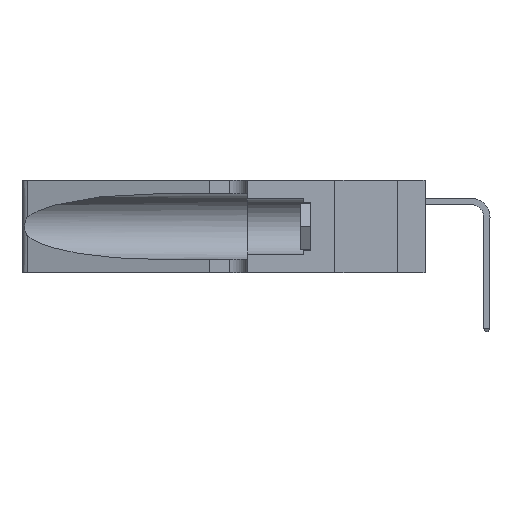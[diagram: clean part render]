
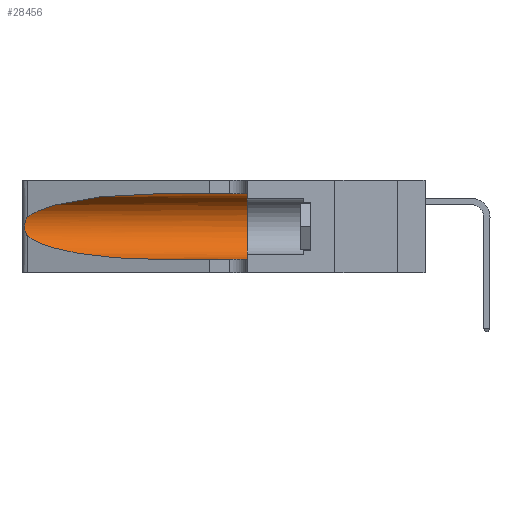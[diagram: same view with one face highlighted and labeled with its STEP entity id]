
A CAD part, left-side view. The second image highlights one B-rep face of the part: STEP entity #28456.
In plain terms, the highlighted cylindrical face has radius 3.308 mm (diameter 6.617 mm), a partial arc.
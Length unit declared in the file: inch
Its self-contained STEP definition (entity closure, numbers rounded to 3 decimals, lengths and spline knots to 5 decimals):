
#971 = CARTESIAN_POINT ( 'NONE',  ( 0.25787, 1.23484, 0.2124 ) ) ;
#2209 = CARTESIAN_POINT ( 'NONE',  ( 0.1305, 0.72297, 0.31525 ) ) ;
#2385 = B_SPLINE_CURVE_WITH_KNOTS ( 'NONE', 3,
 ( #15900, #33694, #18909, #971, #21850, #4006, #24819, #6992, #27801, #10040, #30830, #13051, #33829, #16030 ),
 .UNSPECIFIED., .F., .F.,
 ( 4, 2, 2, 2, 2, 2, 4 ),
 ( 0., 0.00027, 0.00053, 0.00107, 0.0016, 0.00187, 0.00214 ),
 .UNSPECIFIED. ) ;
#4006 = CARTESIAN_POINT ( 'NONE',  ( 0.26018, 1.23835, 0.19895 ) ) ;
#4031 = CYLINDRICAL_SURFACE ( 'NONE', #36166, 0.13025 ) ;
#4401 = CARTESIAN_POINT ( 'NONE',  ( 0.1305, 1.61858, 0.31525 ) ) ;
#5489 = VECTOR ( 'NONE', #11090, 39.37008 ) ;
#5728 = CARTESIAN_POINT ( 'NONE',  ( 0.1305, 0.35, 0.31525 ) ) ;
#6696 = CARTESIAN_POINT ( 'NONE',  ( 0.25487, 1.22718, 0.14631 ) ) ;
#6992 = CARTESIAN_POINT ( 'NONE',  ( 0.26075, 1.23896, 0.178 ) ) ;
#7516 = CARTESIAN_POINT ( 'NONE',  ( 0.18966, 0.96281, 0.31525 ) ) ;
#8796 = ORIENTED_EDGE ( 'NONE', *, *, #12495, .F. ) ;
#9128 = ORIENTED_EDGE ( 'NONE', *, *, #11429, .T. ) ;
#9142 = DIRECTION ( 'NONE',  ( 0., 1., 0. ) ) ;
#9740 = CARTESIAN_POINT ( 'NONE',  ( 0.2373, 1.15595, 0.08982 ) ) ;
#10040 = CARTESIAN_POINT ( 'NONE',  ( 0.25856, 1.23593, 0.16098 ) ) ;
#10431 = ORIENTED_EDGE ( 'NONE', *, *, #27737, .T. ) ;
#11090 = DIRECTION ( 'NONE',  ( 0., -1., 0. ) ) ;
#11429 = EDGE_CURVE ( 'NONE', #23252, #27129, #22519, .T. ) ;
#12495 = EDGE_CURVE ( 'NONE', #16182, #30165, #17047, .T. ) ;
#12679 = CARTESIAN_POINT ( 'NONE',  ( 0.1305, 0.35, 0.05475 ) ) ;
#12764 = CARTESIAN_POINT ( 'NONE',  ( 0.1305, 0.72297, 0.05475 ) ) ;
#13051 = CARTESIAN_POINT ( 'NONE',  ( 0.25639, 1.23186, 0.15144 ) ) ;
#13480 = LINE ( 'NONE', #22896, #5489 ) ;
#13501 = LINE ( 'NONE', #4401, #20459 ) ;
#13576 = CARTESIAN_POINT ( 'NONE',  ( 0.1305, 0.72297, 0.31525 ) ) ;
#14316 = DIRECTION ( 'NONE',  ( 0., -1., 0. ) ) ;
#15900 = CARTESIAN_POINT ( 'NONE',  ( 0.25487, 1.22718, 0.22369 ) ) ;
#16030 = CARTESIAN_POINT ( 'NONE',  ( 0.25487, 1.22718, 0.14631 ) ) ;
#16182 = VERTEX_POINT ( 'NONE', #5728 ) ;
#16577 = EDGE_CURVE ( 'NONE', #23252, #16182, #13501, .T. ) ;
#17047 = CIRCLE ( 'NONE', #26182, 0.13025 ) ;
#18909 = CARTESIAN_POINT ( 'NONE',  ( 0.25639, 1.23184, 0.21858 ) ) ;
#20259 = VERTEX_POINT ( 'NONE', #22179 ) ;
#20459 = VECTOR ( 'NONE', #28189, 39.37008 ) ;
#20836 = FACE_OUTER_BOUND ( 'NONE', #25506, .T. ) ;
#21850 = CARTESIAN_POINT ( 'NONE',  ( 0.25854, 1.2359, 0.20912 ) ) ;
#22179 = CARTESIAN_POINT ( 'NONE',  ( 0.1305, 0.72297, 0.05475 ) ) ;
#22519 =( BOUNDED_CURVE ( )  B_SPLINE_CURVE ( 3, ( #13576, #7516, #25333, #34333 ),
 .UNSPECIFIED., .F., .F. ) 
 B_SPLINE_CURVE_WITH_KNOTS ( ( 4, 4 ),
 ( 1.5708, 2.84003 ),
 .UNSPECIFIED. ) 
 CURVE ( )  GEOMETRIC_REPRESENTATION_ITEM ( )  RATIONAL_B_SPLINE_CURVE ( ( 1., 0.87, 0.87, 1. ) ) 
 REPRESENTATION_ITEM ( '' )  );
#22896 = CARTESIAN_POINT ( 'NONE',  ( 0.1305, 1.61858, 0.05475 ) ) ;
#23188 =( BOUNDED_CURVE ( )  B_SPLINE_CURVE ( 3, ( #6696, #9740, #30521, #12764 ),
 .UNSPECIFIED., .F., .F. ) 
 B_SPLINE_CURVE_WITH_KNOTS ( ( 4, 4 ),
 ( 3.44316, 4.71239 ),
 .UNSPECIFIED. ) 
 CURVE ( )  GEOMETRIC_REPRESENTATION_ITEM ( )  RATIONAL_B_SPLINE_CURVE ( ( 1., 0.87, 0.87, 1. ) ) 
 REPRESENTATION_ITEM ( '' )  );
#23252 = VERTEX_POINT ( 'NONE', #2209 ) ;
#23582 = EDGE_CURVE ( 'NONE', #32000, #20259, #23188, .T. ) ;
#24819 = CARTESIAN_POINT ( 'NONE',  ( 0.26075, 1.23896, 0.19203 ) ) ;
#25007 = EDGE_CURVE ( 'NONE', #27129, #32000, #2385, .T. ) ;
#25333 = CARTESIAN_POINT ( 'NONE',  ( 0.2373, 1.15595, 0.28018 ) ) ;
#25506 = EDGE_LOOP ( 'NONE', ( #9128, #30697, #36045, #10431, #8796, #31863 ) ) ;
#26083 = CARTESIAN_POINT ( 'NONE',  ( 0.1305, 1.61858, 0.185 ) ) ;
#26182 = AXIS2_PLACEMENT_3D ( 'NONE', #26925, #9142, #29917 ) ;
#26925 = CARTESIAN_POINT ( 'NONE',  ( 0.1305, 0.35, 0.185 ) ) ;
#27129 = VERTEX_POINT ( 'NONE', #29013 ) ;
#27737 = EDGE_CURVE ( 'NONE', #20259, #30165, #13480, .T. ) ;
#27801 = CARTESIAN_POINT ( 'NONE',  ( 0.26017, 1.23833, 0.17102 ) ) ;
#28189 = DIRECTION ( 'NONE',  ( 0., -1., 0. ) ) ;
#28456 = ADVANCED_FACE ( 'NONE', ( #20836 ), #4031, .F. ) ;
#29013 = CARTESIAN_POINT ( 'NONE',  ( 0.25487, 1.22718, 0.22369 ) ) ;
#29054 = DIRECTION ( 'NONE',  ( 0., 0., -1. ) ) ;
#29917 = DIRECTION ( 'NONE',  ( 0., 0., 1. ) ) ;
#30165 = VERTEX_POINT ( 'NONE', #12679 ) ;
#30521 = CARTESIAN_POINT ( 'NONE',  ( 0.18966, 0.96281, 0.05475 ) ) ;
#30697 = ORIENTED_EDGE ( 'NONE', *, *, #25007, .T. ) ;
#30830 = CARTESIAN_POINT ( 'NONE',  ( 0.25789, 1.23486, 0.15765 ) ) ;
#31863 = ORIENTED_EDGE ( 'NONE', *, *, #16577, .F. ) ;
#32000 = VERTEX_POINT ( 'NONE', #36552 ) ;
#33694 = CARTESIAN_POINT ( 'NONE',  ( 0.25555, 1.22994, 0.2215 ) ) ;
#33829 = CARTESIAN_POINT ( 'NONE',  ( 0.25555, 1.22993, 0.14849 ) ) ;
#34333 = CARTESIAN_POINT ( 'NONE',  ( 0.25487, 1.22718, 0.22369 ) ) ;
#36045 = ORIENTED_EDGE ( 'NONE', *, *, #23582, .T. ) ;
#36166 = AXIS2_PLACEMENT_3D ( 'NONE', #26083, #14316, #29054 ) ;
#36552 = CARTESIAN_POINT ( 'NONE',  ( 0.25487, 1.22718, 0.14631 ) ) ;
